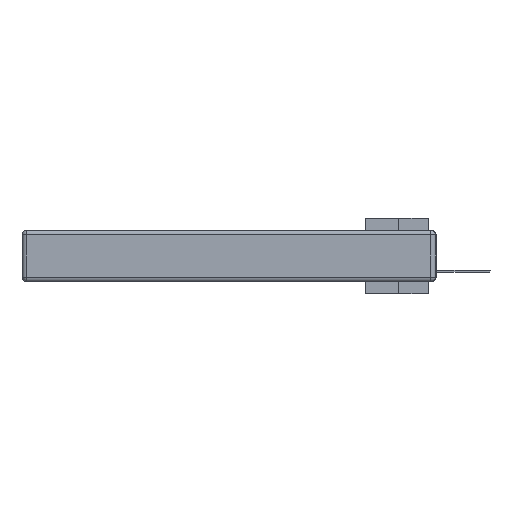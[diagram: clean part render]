
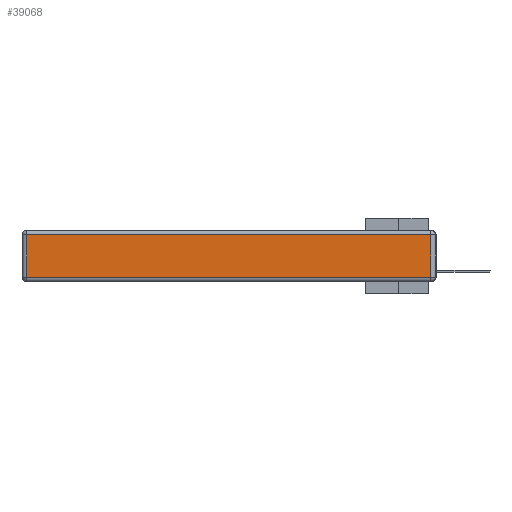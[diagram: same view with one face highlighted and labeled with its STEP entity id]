
A CAD part, left-side view. The second image highlights one B-rep face of the part: STEP entity #39068.
In plain terms, the highlighted planar face has unit normal (-1, 0, 0).
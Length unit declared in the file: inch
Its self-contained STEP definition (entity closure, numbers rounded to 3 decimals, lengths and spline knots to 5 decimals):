
#512 = VERTEX_POINT ( 'NONE', #12112 ) ;
#1024 = DIRECTION ( 'NONE',  ( 0., 0., 1. ) ) ;
#1071 = DIRECTION ( 'NONE',  ( -1., 0., 0. ) ) ;
#2051 = EDGE_LOOP ( 'NONE', ( #5824, #23710, #22980, #17786 ) ) ;
#3706 = EDGE_CURVE ( 'NONE', #24062, #35107, #23519, .T. ) ;
#5371 = VECTOR ( 'NONE', #32918, 39.37008 ) ;
#5824 = ORIENTED_EDGE ( 'NONE', *, *, #12635, .T. ) ;
#7643 = CARTESIAN_POINT ( 'NONE',  ( 0., 2.75, -0.03 ) ) ;
#9016 = CARTESIAN_POINT ( 'NONE',  ( 0., 0.03, -0.343 ) ) ;
#10613 = VECTOR ( 'NONE', #21366, 39.37008 ) ;
#11785 = VECTOR ( 'NONE', #1024, 39.37008 ) ;
#12010 = CARTESIAN_POINT ( 'NONE',  ( 0., 0., -0.313 ) ) ;
#12112 = CARTESIAN_POINT ( 'NONE',  ( 0., 2.72, -0.313 ) ) ;
#12635 = EDGE_CURVE ( 'NONE', #512, #30310, #27488, .T. ) ;
#17786 = ORIENTED_EDGE ( 'NONE', *, *, #36938, .T. ) ;
#18394 = LINE ( 'NONE', #9016, #11785 ) ;
#21366 = DIRECTION ( 'NONE',  ( 0., -1., 0. ) ) ;
#22576 = CARTESIAN_POINT ( 'NONE',  ( 0., 2.72, -0.03 ) ) ;
#22980 = ORIENTED_EDGE ( 'NONE', *, *, #3706, .T. ) ;
#23519 = LINE ( 'NONE', #7643, #28460 ) ;
#23593 = AXIS2_PLACEMENT_3D ( 'NONE', #24966, #1071, #35045 ) ;
#23710 = ORIENTED_EDGE ( 'NONE', *, *, #37597, .T. ) ;
#23763 = CARTESIAN_POINT ( 'NONE',  ( 0., 2.72, -0.343 ) ) ;
#24062 = VERTEX_POINT ( 'NONE', #39173 ) ;
#24966 = CARTESIAN_POINT ( 'NONE',  ( 0., 0., -0.343 ) ) ;
#27488 = LINE ( 'NONE', #12010, #10613 ) ;
#28460 = VECTOR ( 'NONE', #35912, 39.37008 ) ;
#28777 = FACE_OUTER_BOUND ( 'NONE', #2051, .T. ) ;
#30310 = VERTEX_POINT ( 'NONE', #31031 ) ;
#31031 = CARTESIAN_POINT ( 'NONE',  ( 0., 0.03, -0.313 ) ) ;
#32918 = DIRECTION ( 'NONE',  ( 0., 0., -1. ) ) ;
#35045 = DIRECTION ( 'NONE',  ( 0., 0., 1. ) ) ;
#35107 = VERTEX_POINT ( 'NONE', #22576 ) ;
#35252 = PLANE ( 'NONE',  #23593 ) ;
#35912 = DIRECTION ( 'NONE',  ( 0., 1., 0. ) ) ;
#36741 = LINE ( 'NONE', #23763, #5371 ) ;
#36938 = EDGE_CURVE ( 'NONE', #35107, #512, #36741, .T. ) ;
#37597 = EDGE_CURVE ( 'NONE', #30310, #24062, #18394, .T. ) ;
#39068 = ADVANCED_FACE ( 'NONE', ( #28777 ), #35252, .T. ) ;
#39173 = CARTESIAN_POINT ( 'NONE',  ( 0., 0.03, -0.03 ) ) ;
